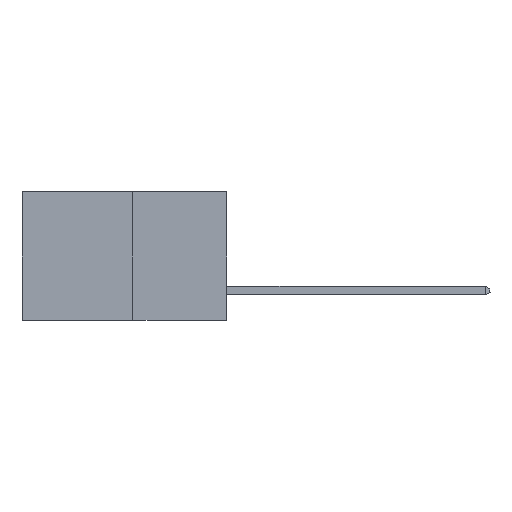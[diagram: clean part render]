
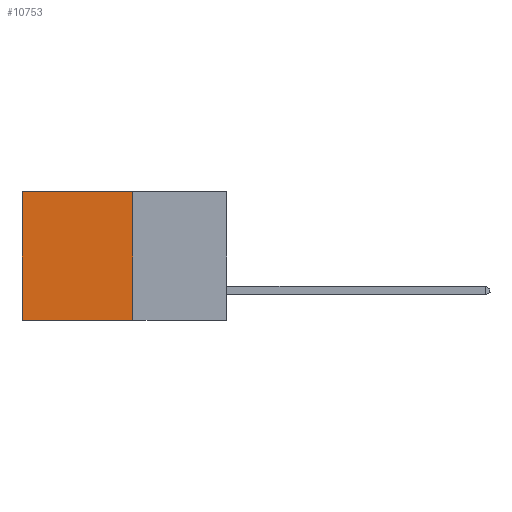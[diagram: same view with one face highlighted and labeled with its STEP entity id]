
A CAD part, left-side view. The second image highlights one B-rep face of the part: STEP entity #10753.
In plain terms, the highlighted planar face has unit normal (-1, 0, 0).
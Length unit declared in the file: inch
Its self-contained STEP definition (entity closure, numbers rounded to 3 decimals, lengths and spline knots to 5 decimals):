
#829 = VERTEX_POINT ( 'NONE', #6239 ) ;
#1130 = LINE ( 'NONE', #11706, #8338 ) ;
#1270 = EDGE_CURVE ( 'NONE', #9157, #11173, #1130, .T. ) ;
#1403 = EDGE_CURVE ( 'NONE', #9157, #5310, #5267, .T. ) ;
#1522 = DIRECTION ( 'NONE',  ( 0., 0., -1. ) ) ;
#1637 = CARTESIAN_POINT ( 'NONE',  ( 0.277, 0.27, 0. ) ) ;
#2531 = CARTESIAN_POINT ( 'NONE',  ( 0.277, 0.27, -0.37 ) ) ;
#2858 = CARTESIAN_POINT ( 'NONE',  ( 0.277, 0.27, -0.37 ) ) ;
#3372 = CARTESIAN_POINT ( 'NONE',  ( 0.277, 0.59, -0.37 ) ) ;
#3434 = AXIS2_PLACEMENT_3D ( 'NONE', #2858, #10332, #4765 ) ;
#4342 = FACE_OUTER_BOUND ( 'NONE', #10600, .T. ) ;
#4433 = DIRECTION ( 'NONE',  ( 0., 1., 0. ) ) ;
#4651 = VECTOR ( 'NONE', #1522, 39.37008 ) ;
#4765 = DIRECTION ( 'NONE',  ( 0., 0., -1. ) ) ;
#5267 = LINE ( 'NONE', #1637, #9628 ) ;
#5310 = VERTEX_POINT ( 'NONE', #10107 ) ;
#5906 = EDGE_CURVE ( 'NONE', #5310, #829, #9603, .T. ) ;
#6239 = CARTESIAN_POINT ( 'NONE',  ( 0.277, 0.59, -0.37 ) ) ;
#6540 = ORIENTED_EDGE ( 'NONE', *, *, #1270, .F. ) ;
#6916 = CARTESIAN_POINT ( 'NONE',  ( 0.277, 0.27, 0. ) ) ;
#7189 = CARTESIAN_POINT ( 'NONE',  ( 0.277, 0.27, -0.37 ) ) ;
#8100 = DIRECTION ( 'NONE',  ( 0., 1., 0. ) ) ;
#8160 = ORIENTED_EDGE ( 'NONE', *, *, #11952, .F. ) ;
#8338 = VECTOR ( 'NONE', #10787, 39.37008 ) ;
#8561 = VECTOR ( 'NONE', #8100, 39.37008 ) ;
#8815 = ORIENTED_EDGE ( 'NONE', *, *, #1403, .T. ) ;
#9157 = VERTEX_POINT ( 'NONE', #6916 ) ;
#9402 = PLANE ( 'NONE',  #3434 ) ;
#9603 = LINE ( 'NONE', #3372, #4651 ) ;
#9628 = VECTOR ( 'NONE', #4433, 39.37008 ) ;
#9650 = ORIENTED_EDGE ( 'NONE', *, *, #5906, .T. ) ;
#10107 = CARTESIAN_POINT ( 'NONE',  ( 0.277, 0.59, 0. ) ) ;
#10332 = DIRECTION ( 'NONE',  ( 1., 0., 0. ) ) ;
#10600 = EDGE_LOOP ( 'NONE', ( #9650, #8160, #6540, #8815 ) ) ;
#10753 = ADVANCED_FACE ( 'NONE', ( #4342 ), #9402, .F. ) ;
#10787 = DIRECTION ( 'NONE',  ( 0., 0., -1. ) ) ;
#11173 = VERTEX_POINT ( 'NONE', #2531 ) ;
#11293 = LINE ( 'NONE', #7189, #8561 ) ;
#11706 = CARTESIAN_POINT ( 'NONE',  ( 0.277, 0.27, -0.37 ) ) ;
#11952 = EDGE_CURVE ( 'NONE', #11173, #829, #11293, .T. ) ;
